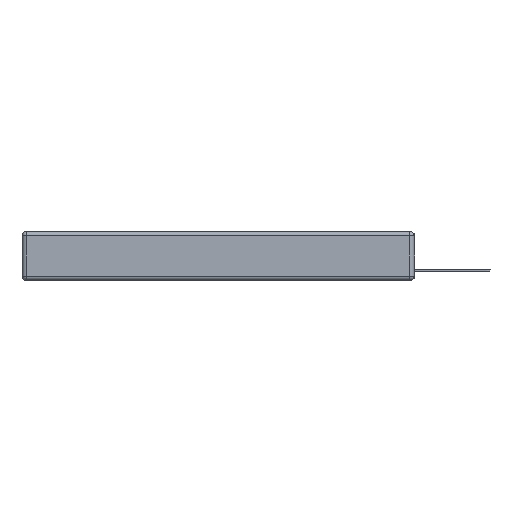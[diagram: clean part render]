
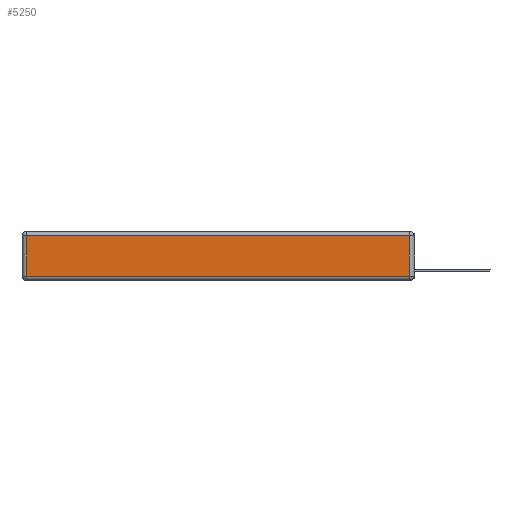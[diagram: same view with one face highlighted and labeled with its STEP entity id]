
A CAD part, left-side view. The second image highlights one B-rep face of the part: STEP entity #5250.
In plain terms, the highlighted planar face has unit normal (-1, 0, 0).
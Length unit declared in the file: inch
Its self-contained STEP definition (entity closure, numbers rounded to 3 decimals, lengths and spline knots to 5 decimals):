
#10 = VERTEX_POINT ( 'NONE', #334 ) ;
#92 = LINE ( 'NONE', #3480, #1066 ) ;
#134 = AXIS2_PLACEMENT_3D ( 'NONE', #11190, #4790, #11143 ) ;
#334 = CARTESIAN_POINT ( 'NONE',  ( 0., 0.03, -0.03 ) ) ;
#458 = VECTOR ( 'NONE', #7890, 39.37008 ) ;
#1066 = VECTOR ( 'NONE', #2345, 39.37008 ) ;
#1250 = EDGE_CURVE ( 'NONE', #2499, #15330, #13279, .T. ) ;
#2345 = DIRECTION ( 'NONE',  ( 0., 1., 0. ) ) ;
#2499 = VERTEX_POINT ( 'NONE', #5976 ) ;
#3480 = CARTESIAN_POINT ( 'NONE',  ( 0., 2.75, -0.03 ) ) ;
#3685 = CARTESIAN_POINT ( 'NONE',  ( 0., 0., -0.313 ) ) ;
#4462 = ORIENTED_EDGE ( 'NONE', *, *, #1250, .T. ) ;
#4790 = DIRECTION ( 'NONE',  ( -1., 0., 0. ) ) ;
#5102 = VECTOR ( 'NONE', #13652, 39.37008 ) ;
#5250 = ADVANCED_FACE ( 'NONE', ( #10435 ), #6111, .T. ) ;
#5786 = EDGE_CURVE ( 'NONE', #10, #5882, #92, .T. ) ;
#5882 = VERTEX_POINT ( 'NONE', #15589 ) ;
#5976 = CARTESIAN_POINT ( 'NONE',  ( 0., 2.72, -0.313 ) ) ;
#6111 = PLANE ( 'NONE',  #134 ) ;
#6134 = CARTESIAN_POINT ( 'NONE',  ( 0., 0.03, -0.343 ) ) ;
#6684 = EDGE_CURVE ( 'NONE', #5882, #2499, #14741, .T. ) ;
#7729 = EDGE_CURVE ( 'NONE', #15330, #10, #8116, .T. ) ;
#7890 = DIRECTION ( 'NONE',  ( 0., 0., -1. ) ) ;
#8116 = LINE ( 'NONE', #6134, #15861 ) ;
#9482 = CARTESIAN_POINT ( 'NONE',  ( 0., 0.03, -0.313 ) ) ;
#9646 = EDGE_LOOP ( 'NONE', ( #4462, #12825, #14194, #10379 ) ) ;
#10379 = ORIENTED_EDGE ( 'NONE', *, *, #6684, .T. ) ;
#10435 = FACE_OUTER_BOUND ( 'NONE', #9646, .T. ) ;
#10471 = DIRECTION ( 'NONE',  ( 0., 0., 1. ) ) ;
#11143 = DIRECTION ( 'NONE',  ( 0., 0., 1. ) ) ;
#11190 = CARTESIAN_POINT ( 'NONE',  ( 0., 0., -0.343 ) ) ;
#12825 = ORIENTED_EDGE ( 'NONE', *, *, #7729, .T. ) ;
#13279 = LINE ( 'NONE', #3685, #5102 ) ;
#13652 = DIRECTION ( 'NONE',  ( 0., -1., 0. ) ) ;
#14194 = ORIENTED_EDGE ( 'NONE', *, *, #5786, .T. ) ;
#14741 = LINE ( 'NONE', #15649, #458 ) ;
#15330 = VERTEX_POINT ( 'NONE', #9482 ) ;
#15589 = CARTESIAN_POINT ( 'NONE',  ( 0., 2.72, -0.03 ) ) ;
#15649 = CARTESIAN_POINT ( 'NONE',  ( 0., 2.72, -0.343 ) ) ;
#15861 = VECTOR ( 'NONE', #10471, 39.37008 ) ;
